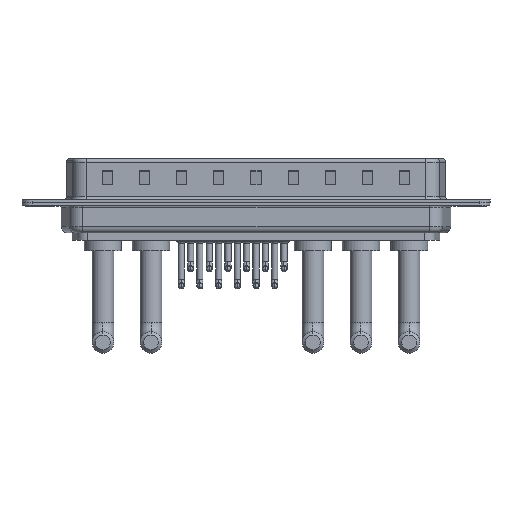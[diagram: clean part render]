
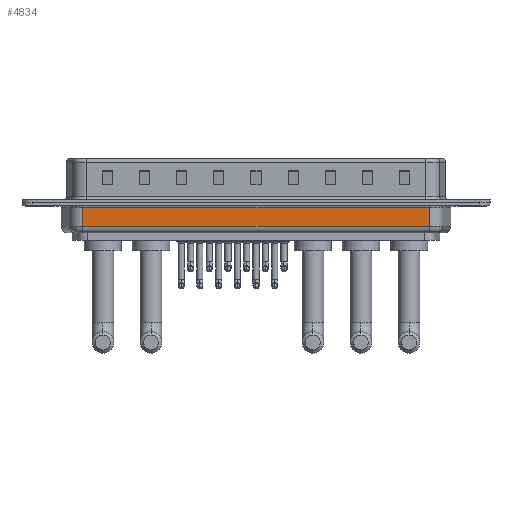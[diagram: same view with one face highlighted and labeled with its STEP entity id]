
A CAD part, front view. The second image highlights one B-rep face of the part: STEP entity #4834.
In plain terms, the highlighted planar face has unit normal (0, -1, 0).
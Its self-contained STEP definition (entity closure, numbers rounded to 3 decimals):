
#466 = DIRECTION ( 'NONE',  ( 1., 0., 0. ) ) ;
#1776 = DIRECTION ( 'NONE',  ( 0., 0., 1. ) ) ;
#2052 = ORIENTED_EDGE ( 'NONE', *, *, #14418, .T. ) ;
#2257 = EDGE_CURVE ( 'NONE', #4675, #15043, #23605, .T. ) ;
#3257 = CARTESIAN_POINT ( 'NONE',  ( 6.031, -5.35, -3.5 ) ) ;
#3290 = ORIENTED_EDGE ( 'NONE', *, *, #3343, .T. ) ;
#3343 = EDGE_CURVE ( 'NONE', #4675, #20319, #19020, .T. ) ;
#4675 = VERTEX_POINT ( 'NONE', #3257 ) ;
#4834 = ADVANCED_FACE ( 'NONE', ( #14435 ), #21801, .F. ) ;
#6360 = ORIENTED_EDGE ( 'NONE', *, *, #2257, .F. ) ;
#6797 = DIRECTION ( 'NONE',  ( 0., 0., 1. ) ) ;
#7220 = CARTESIAN_POINT ( 'NONE',  ( 6.031, -5.35, -4.5 ) ) ;
#8584 = VECTOR ( 'NONE', #6797, 1000. ) ;
#8729 = VECTOR ( 'NONE', #466, 1000. ) ;
#8975 = CARTESIAN_POINT ( 'NONE',  ( 57.469, -5.35, -0.65 ) ) ;
#8999 = CARTESIAN_POINT ( 'NONE',  ( 6.031, -5.35, -4.5 ) ) ;
#10112 = CARTESIAN_POINT ( 'NONE',  ( 6.031, -5.35, -0.65 ) ) ;
#11771 = CARTESIAN_POINT ( 'NONE',  ( 6.031, -5.35, -3.5 ) ) ;
#12620 = DIRECTION ( 'NONE',  ( 0., 1., 0. ) ) ;
#13848 = VERTEX_POINT ( 'NONE', #8975 ) ;
#13996 = CARTESIAN_POINT ( 'NONE',  ( 57.469, -5.35, -4.5 ) ) ;
#14148 = VECTOR ( 'NONE', #1776, 1000. ) ;
#14188 = EDGE_CURVE ( 'NONE', #20319, #13848, #23306, .T. ) ;
#14418 = EDGE_CURVE ( 'NONE', #13848, #15043, #19509, .T. ) ;
#14435 = FACE_OUTER_BOUND ( 'NONE', #22646, .T. ) ;
#15043 = VERTEX_POINT ( 'NONE', #21259 ) ;
#16803 = CARTESIAN_POINT ( 'NONE',  ( 57.469, -5.35, -3.5 ) ) ;
#19020 = LINE ( 'NONE', #11771, #8729 ) ;
#19509 = LINE ( 'NONE', #10112, #20530 ) ;
#20319 = VERTEX_POINT ( 'NONE', #16803 ) ;
#20530 = VECTOR ( 'NONE', #23384, 1000. ) ;
#21063 = ORIENTED_EDGE ( 'NONE', *, *, #14188, .T. ) ;
#21121 = AXIS2_PLACEMENT_3D ( 'NONE', #7220, #12620, #22168 ) ;
#21259 = CARTESIAN_POINT ( 'NONE',  ( 6.031, -5.35, -0.65 ) ) ;
#21801 = PLANE ( 'NONE',  #21121 ) ;
#22168 = DIRECTION ( 'NONE',  ( -1., 0., 0. ) ) ;
#22646 = EDGE_LOOP ( 'NONE', ( #6360, #3290, #21063, #2052 ) ) ;
#23306 = LINE ( 'NONE', #13996, #8584 ) ;
#23384 = DIRECTION ( 'NONE',  ( -1., 0., 0. ) ) ;
#23605 = LINE ( 'NONE', #8999, #14148 ) ;
